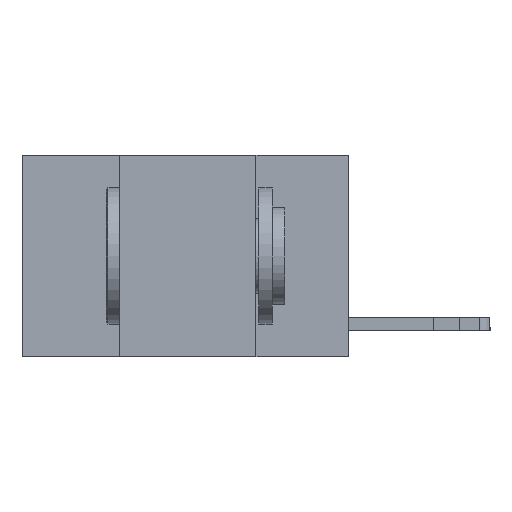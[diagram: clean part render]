
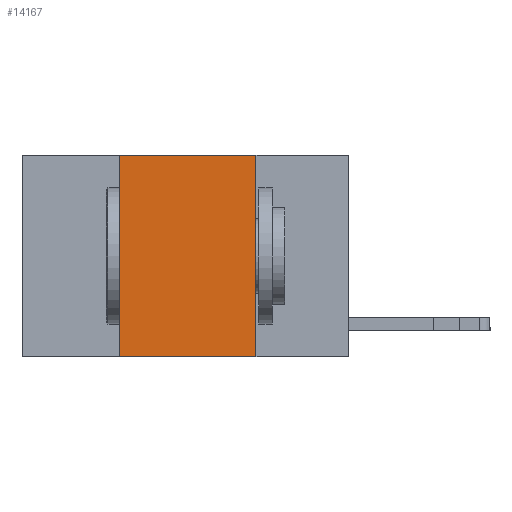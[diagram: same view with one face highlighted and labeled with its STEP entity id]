
A CAD part, left-side view. The second image highlights one B-rep face of the part: STEP entity #14167.
In plain terms, the highlighted planar face has unit normal (-1, 0, 0).
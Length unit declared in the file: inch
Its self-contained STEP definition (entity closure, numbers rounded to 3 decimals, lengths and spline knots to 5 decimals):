
#19 = DIRECTION ( 'NONE',  ( 0., -1., 0. ) ) ;
#1331 = VECTOR ( 'NONE', #14551, 39.37008 ) ;
#1542 = EDGE_CURVE ( 'NONE', #10400, #8071, #19774, .T. ) ;
#1689 = VERTEX_POINT ( 'NONE', #13901 ) ;
#4345 = LINE ( 'NONE', #12255, #18730 ) ;
#4479 = EDGE_LOOP ( 'NONE', ( #9606, #11166, #19348, #8052 ) ) ;
#4630 = EDGE_CURVE ( 'NONE', #5208, #1689, #9676, .T. ) ;
#5208 = VERTEX_POINT ( 'NONE', #5956 ) ;
#5424 = PLANE ( 'NONE',  #8963 ) ;
#5956 = CARTESIAN_POINT ( 'NONE',  ( 0., 0.42, 0. ) ) ;
#5962 = CARTESIAN_POINT ( 'NONE',  ( 0., 0.42, -0.37 ) ) ;
#6423 = CARTESIAN_POINT ( 'NONE',  ( 0., 0.6, 0. ) ) ;
#6817 = CARTESIAN_POINT ( 'NONE',  ( 0., 0.17, -0.37 ) ) ;
#7772 = EDGE_CURVE ( 'NONE', #10400, #5208, #4345, .T. ) ;
#7873 = VECTOR ( 'NONE', #19, 39.37008 ) ;
#8052 = ORIENTED_EDGE ( 'NONE', *, *, #1542, .T. ) ;
#8071 = VERTEX_POINT ( 'NONE', #6817 ) ;
#8963 = AXIS2_PLACEMENT_3D ( 'NONE', #12033, #18644, #10413 ) ;
#9606 = ORIENTED_EDGE ( 'NONE', *, *, #13813, .F. ) ;
#9676 = LINE ( 'NONE', #6423, #10469 ) ;
#10400 = VERTEX_POINT ( 'NONE', #5962 ) ;
#10413 = DIRECTION ( 'NONE',  ( 0., 0., -1. ) ) ;
#10469 = VECTOR ( 'NONE', #14774, 39.37008 ) ;
#10568 = LINE ( 'NONE', #14331, #1331 ) ;
#11166 = ORIENTED_EDGE ( 'NONE', *, *, #4630, .F. ) ;
#12033 = CARTESIAN_POINT ( 'NONE',  ( 0., 0.6, 0. ) ) ;
#12255 = CARTESIAN_POINT ( 'NONE',  ( 0., 0.42, 0. ) ) ;
#13813 = EDGE_CURVE ( 'NONE', #1689, #8071, #10568, .T. ) ;
#13901 = CARTESIAN_POINT ( 'NONE',  ( 0., 0.17, 0. ) ) ;
#14167 = ADVANCED_FACE ( 'NONE', ( #20283 ), #5424, .F. ) ;
#14331 = CARTESIAN_POINT ( 'NONE',  ( 0., 0.17, 0. ) ) ;
#14551 = DIRECTION ( 'NONE',  ( 0., 0., -1. ) ) ;
#14774 = DIRECTION ( 'NONE',  ( 0., -1., 0. ) ) ;
#17439 = DIRECTION ( 'NONE',  ( 0., 0., 1. ) ) ;
#18128 = CARTESIAN_POINT ( 'NONE',  ( 0., 0.6, -0.37 ) ) ;
#18644 = DIRECTION ( 'NONE',  ( 1., 0., 0. ) ) ;
#18730 = VECTOR ( 'NONE', #17439, 39.37008 ) ;
#19348 = ORIENTED_EDGE ( 'NONE', *, *, #7772, .F. ) ;
#19774 = LINE ( 'NONE', #18128, #7873 ) ;
#20283 = FACE_OUTER_BOUND ( 'NONE', #4479, .T. ) ;
